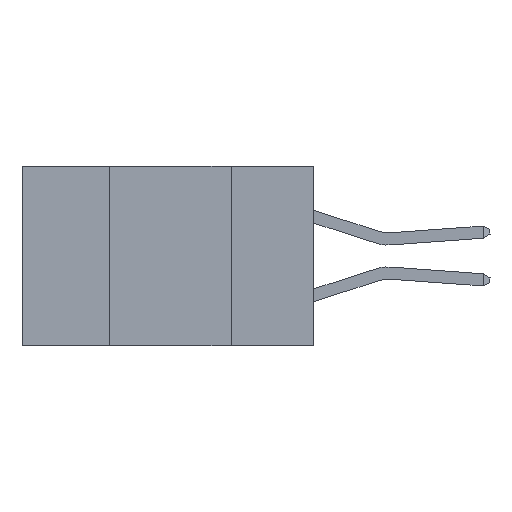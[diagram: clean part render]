
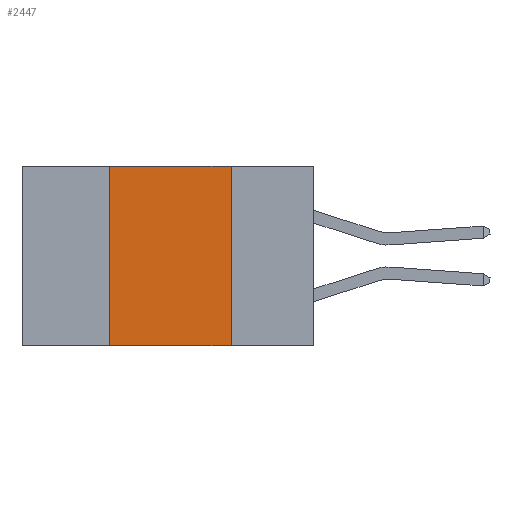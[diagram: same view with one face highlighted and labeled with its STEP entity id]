
A CAD part, left-side view. The second image highlights one B-rep face of the part: STEP entity #2447.
In plain terms, the highlighted planar face has unit normal (-1, 0, 0).
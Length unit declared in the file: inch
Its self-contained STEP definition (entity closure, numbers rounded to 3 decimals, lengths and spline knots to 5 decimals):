
#70 = LINE ( 'NONE', #22891, #5484 ) ;
#863 = CARTESIAN_POINT ( 'NONE',  ( 0., 0.17, 0. ) ) ;
#1525 = VERTEX_POINT ( 'NONE', #15739 ) ;
#1634 = LINE ( 'NONE', #14354, #7605 ) ;
#2447 = ADVANCED_FACE ( 'NONE', ( #13880 ), #6165, .F. ) ;
#2639 = DIRECTION ( 'NONE',  ( 0., 0., -1. ) ) ;
#4117 = CARTESIAN_POINT ( 'NONE',  ( 0., 0.42, -0.37 ) ) ;
#5484 = VECTOR ( 'NONE', #11882, 39.37008 ) ;
#6165 = PLANE ( 'NONE',  #23774 ) ;
#6285 = VERTEX_POINT ( 'NONE', #23495 ) ;
#7304 = VECTOR ( 'NONE', #8978, 39.37008 ) ;
#7605 = VECTOR ( 'NONE', #2639, 39.37008 ) ;
#8117 = DIRECTION ( 'NONE',  ( 1., 0., 0. ) ) ;
#8688 = ORIENTED_EDGE ( 'NONE', *, *, #22264, .F. ) ;
#8978 = DIRECTION ( 'NONE',  ( 0., 0., 1. ) ) ;
#11659 = VECTOR ( 'NONE', #18371, 39.37008 ) ;
#11882 = DIRECTION ( 'NONE',  ( 0., -1., 0. ) ) ;
#12422 = EDGE_CURVE ( 'NONE', #12983, #1525, #70, .T. ) ;
#12983 = VERTEX_POINT ( 'NONE', #4117 ) ;
#13011 = LINE ( 'NONE', #18347, #7304 ) ;
#13196 = ORIENTED_EDGE ( 'NONE', *, *, #20168, .F. ) ;
#13324 = EDGE_CURVE ( 'NONE', #6285, #16239, #22606, .T. ) ;
#13642 = EDGE_LOOP ( 'NONE', ( #13196, #22911, #8688, #24042 ) ) ;
#13880 = FACE_OUTER_BOUND ( 'NONE', #13642, .T. ) ;
#14354 = CARTESIAN_POINT ( 'NONE',  ( 0., 0.17, 0. ) ) ;
#15739 = CARTESIAN_POINT ( 'NONE',  ( 0., 0.17, -0.37 ) ) ;
#16239 = VERTEX_POINT ( 'NONE', #863 ) ;
#16523 = CARTESIAN_POINT ( 'NONE',  ( 0., 0.6, 0. ) ) ;
#18347 = CARTESIAN_POINT ( 'NONE',  ( 0., 0.42, 0. ) ) ;
#18371 = DIRECTION ( 'NONE',  ( 0., -1., 0. ) ) ;
#19367 = CARTESIAN_POINT ( 'NONE',  ( 0., 0.6, 0. ) ) ;
#20168 = EDGE_CURVE ( 'NONE', #16239, #1525, #1634, .T. ) ;
#21149 = DIRECTION ( 'NONE',  ( 0., 0., -1. ) ) ;
#22264 = EDGE_CURVE ( 'NONE', #12983, #6285, #13011, .T. ) ;
#22606 = LINE ( 'NONE', #16523, #11659 ) ;
#22891 = CARTESIAN_POINT ( 'NONE',  ( 0., 0.6, -0.37 ) ) ;
#22911 = ORIENTED_EDGE ( 'NONE', *, *, #13324, .F. ) ;
#23495 = CARTESIAN_POINT ( 'NONE',  ( 0., 0.42, 0. ) ) ;
#23774 = AXIS2_PLACEMENT_3D ( 'NONE', #19367, #8117, #21149 ) ;
#24042 = ORIENTED_EDGE ( 'NONE', *, *, #12422, .T. ) ;
